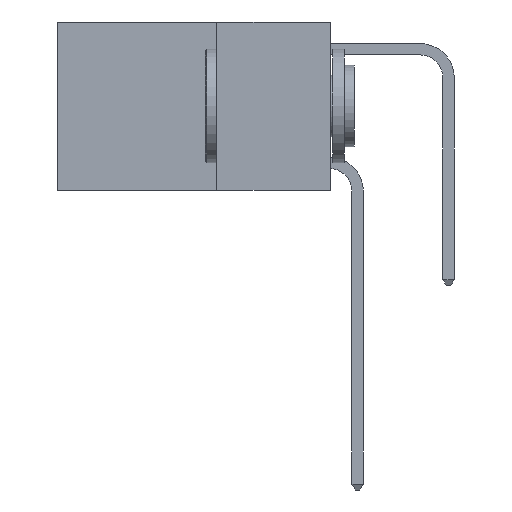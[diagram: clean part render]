
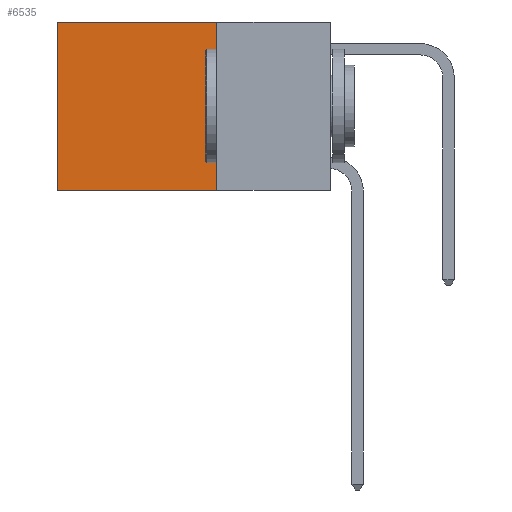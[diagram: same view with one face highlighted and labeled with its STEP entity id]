
A CAD part, left-side view. The second image highlights one B-rep face of the part: STEP entity #6535.
In plain terms, the highlighted planar face has unit normal (-1, 0, 0).
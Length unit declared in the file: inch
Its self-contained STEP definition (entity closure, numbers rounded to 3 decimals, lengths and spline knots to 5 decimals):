
#271 = LINE ( 'NONE', #4794, #10017 ) ;
#374 = EDGE_CURVE ( 'NONE', #1528, #2619, #2384, .T. ) ;
#583 = ORIENTED_EDGE ( 'NONE', *, *, #374, .F. ) ;
#756 = EDGE_LOOP ( 'NONE', ( #4580, #583, #9438, #10401 ) ) ;
#1001 = PLANE ( 'NONE',  #3132 ) ;
#1080 = EDGE_CURVE ( 'NONE', #6433, #5757, #6520, .T. ) ;
#1086 = FACE_OUTER_BOUND ( 'NONE', #756, .T. ) ;
#1528 = VERTEX_POINT ( 'NONE', #3196 ) ;
#1915 = CARTESIAN_POINT ( 'NONE',  ( 0.2625, 0.25, 0. ) ) ;
#2384 = LINE ( 'NONE', #7460, #3566 ) ;
#2619 = VERTEX_POINT ( 'NONE', #9355 ) ;
#2872 = CARTESIAN_POINT ( 'NONE',  ( 0.2625, 0.25, 0. ) ) ;
#3132 = AXIS2_PLACEMENT_3D ( 'NONE', #5195, #9280, #4321 ) ;
#3196 = CARTESIAN_POINT ( 'NONE',  ( 0.2625, 0.25, -0.37 ) ) ;
#3566 = VECTOR ( 'NONE', #5180, 39.37008 ) ;
#3862 = EDGE_CURVE ( 'NONE', #5757, #2619, #271, .T. ) ;
#4321 = DIRECTION ( 'NONE',  ( 0., 0., -1. ) ) ;
#4580 = ORIENTED_EDGE ( 'NONE', *, *, #3862, .T. ) ;
#4794 = CARTESIAN_POINT ( 'NONE',  ( 0.2625, 0.6, 0. ) ) ;
#4939 = CARTESIAN_POINT ( 'NONE',  ( 0.2625, 0.6, 0. ) ) ;
#5144 = VECTOR ( 'NONE', #10673, 39.37008 ) ;
#5180 = DIRECTION ( 'NONE',  ( 0., 1., 0. ) ) ;
#5195 = CARTESIAN_POINT ( 'NONE',  ( 0.2625, 0.25, 0. ) ) ;
#5757 = VERTEX_POINT ( 'NONE', #4939 ) ;
#6114 = DIRECTION ( 'NONE',  ( 0., 0., -1. ) ) ;
#6433 = VERTEX_POINT ( 'NONE', #1915 ) ;
#6520 = LINE ( 'NONE', #9536, #5144 ) ;
#6535 = ADVANCED_FACE ( 'NONE', ( #1086 ), #1001, .F. ) ;
#6746 = LINE ( 'NONE', #2872, #6973 ) ;
#6973 = VECTOR ( 'NONE', #9697, 39.37008 ) ;
#7222 = EDGE_CURVE ( 'NONE', #6433, #1528, #6746, .T. ) ;
#7460 = CARTESIAN_POINT ( 'NONE',  ( 0.2625, 0.25, -0.37 ) ) ;
#9280 = DIRECTION ( 'NONE',  ( 1., 0., 0. ) ) ;
#9355 = CARTESIAN_POINT ( 'NONE',  ( 0.2625, 0.6, -0.37 ) ) ;
#9438 = ORIENTED_EDGE ( 'NONE', *, *, #7222, .F. ) ;
#9536 = CARTESIAN_POINT ( 'NONE',  ( 0.2625, 0.25, 0. ) ) ;
#9697 = DIRECTION ( 'NONE',  ( 0., 0., -1. ) ) ;
#10017 = VECTOR ( 'NONE', #6114, 39.37008 ) ;
#10401 = ORIENTED_EDGE ( 'NONE', *, *, #1080, .T. ) ;
#10673 = DIRECTION ( 'NONE',  ( 0., 1., 0. ) ) ;
